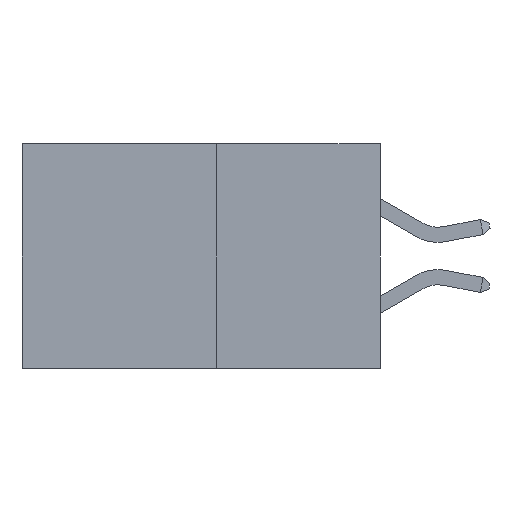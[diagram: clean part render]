
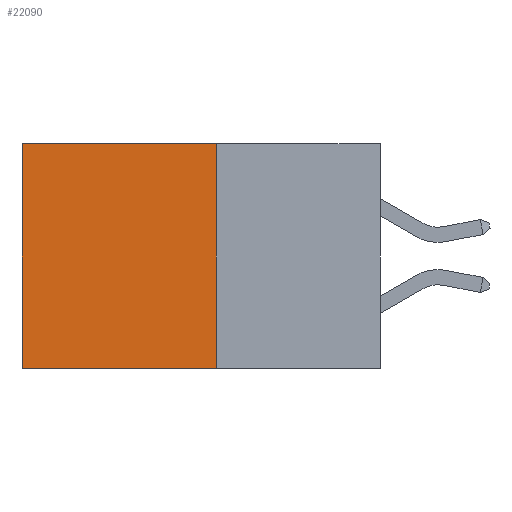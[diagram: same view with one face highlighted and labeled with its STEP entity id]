
A CAD part, left-side view. The second image highlights one B-rep face of the part: STEP entity #22090.
In plain terms, the highlighted planar face has unit normal (-1, 0, 0).
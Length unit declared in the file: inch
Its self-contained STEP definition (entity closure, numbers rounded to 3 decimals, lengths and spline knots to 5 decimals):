
#688 = ORIENTED_EDGE ( 'NONE', *, *, #19879, .F. ) ;
#1265 = ORIENTED_EDGE ( 'NONE', *, *, #25887, .T. ) ;
#1470 = CARTESIAN_POINT ( 'NONE',  ( 0.277, 0.27, -0.37 ) ) ;
#2364 = VECTOR ( 'NONE', #27910, 39.37008 ) ;
#4287 = PLANE ( 'NONE',  #14431 ) ;
#5873 = LINE ( 'NONE', #26368, #26894 ) ;
#5991 = CARTESIAN_POINT ( 'NONE',  ( 0.277, 0.27, -0.37 ) ) ;
#7084 = VERTEX_POINT ( 'NONE', #17497 ) ;
#7709 = CARTESIAN_POINT ( 'NONE',  ( 0.277, 0.27, -0.37 ) ) ;
#12992 = LINE ( 'NONE', #28096, #19492 ) ;
#13066 = ORIENTED_EDGE ( 'NONE', *, *, #34644, .T. ) ;
#14101 = CARTESIAN_POINT ( 'NONE',  ( 0.277, 0.27, 0. ) ) ;
#14388 = DIRECTION ( 'NONE',  ( 0., 1., 0. ) ) ;
#14431 = AXIS2_PLACEMENT_3D ( 'NONE', #1470, #31615, #23535 ) ;
#17497 = CARTESIAN_POINT ( 'NONE',  ( 0.277, 0.59, -0.37 ) ) ;
#19455 = VERTEX_POINT ( 'NONE', #27235 ) ;
#19492 = VECTOR ( 'NONE', #19961, 39.37008 ) ;
#19879 = EDGE_CURVE ( 'NONE', #32671, #7084, #5873, .T. ) ;
#19961 = DIRECTION ( 'NONE',  ( 0., 0., -1. ) ) ;
#22087 = VECTOR ( 'NONE', #14388, 39.37008 ) ;
#22090 = ADVANCED_FACE ( 'NONE', ( #29768 ), #4287, .F. ) ;
#23535 = DIRECTION ( 'NONE',  ( 0., 0., -1. ) ) ;
#24028 = EDGE_CURVE ( 'NONE', #35230, #32671, #30711, .T. ) ;
#25289 = EDGE_LOOP ( 'NONE', ( #1265, #688, #33561, #13066 ) ) ;
#25887 = EDGE_CURVE ( 'NONE', #19455, #7084, #12992, .T. ) ;
#26368 = CARTESIAN_POINT ( 'NONE',  ( 0.277, 0.27, -0.37 ) ) ;
#26894 = VECTOR ( 'NONE', #31860, 39.37008 ) ;
#27235 = CARTESIAN_POINT ( 'NONE',  ( 0.277, 0.59, 0. ) ) ;
#27910 = DIRECTION ( 'NONE',  ( 0., 0., -1. ) ) ;
#28096 = CARTESIAN_POINT ( 'NONE',  ( 0.277, 0.59, -0.37 ) ) ;
#29768 = FACE_OUTER_BOUND ( 'NONE', #25289, .T. ) ;
#30206 = LINE ( 'NONE', #33566, #22087 ) ;
#30711 = LINE ( 'NONE', #5991, #2364 ) ;
#31615 = DIRECTION ( 'NONE',  ( 1., 0., 0. ) ) ;
#31860 = DIRECTION ( 'NONE',  ( 0., 1., 0. ) ) ;
#32671 = VERTEX_POINT ( 'NONE', #7709 ) ;
#33561 = ORIENTED_EDGE ( 'NONE', *, *, #24028, .F. ) ;
#33566 = CARTESIAN_POINT ( 'NONE',  ( 0.277, 0.27, 0. ) ) ;
#34644 = EDGE_CURVE ( 'NONE', #35230, #19455, #30206, .T. ) ;
#35230 = VERTEX_POINT ( 'NONE', #14101 ) ;
